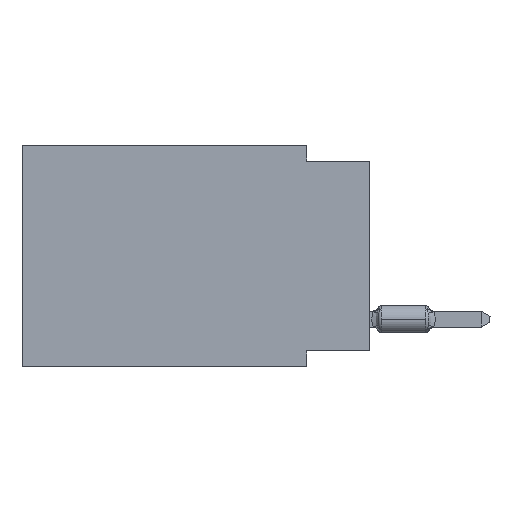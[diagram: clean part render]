
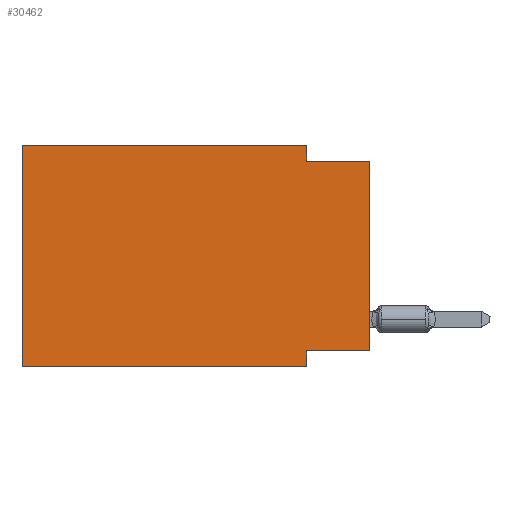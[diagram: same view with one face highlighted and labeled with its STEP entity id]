
A CAD part, left-side view. The second image highlights one B-rep face of the part: STEP entity #30462.
In plain terms, the highlighted planar face has unit normal (-1, 0, 0).
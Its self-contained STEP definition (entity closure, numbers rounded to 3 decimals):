
#1430 = VERTEX_POINT ( 'NONE', #4107 ) ;
#1948 = ORIENTED_EDGE ( 'NONE', *, *, #29080, .F. ) ;
#2856 = ORIENTED_EDGE ( 'NONE', *, *, #14217, .F. ) ;
#3091 = CARTESIAN_POINT ( 'NONE',  ( 0., 2.54, 0. ) ) ;
#3257 = DIRECTION ( 'NONE',  ( 1., 0., 0. ) ) ;
#3844 = VERTEX_POINT ( 'NONE', #28738 ) ;
#4045 = EDGE_CURVE ( 'NONE', #5214, #22583, #24029, .T. ) ;
#4107 = CARTESIAN_POINT ( 'NONE',  ( 0., 2.54, -8.255 ) ) ;
#5006 = DIRECTION ( 'NONE',  ( 0., -1., 0. ) ) ;
#5214 = VERTEX_POINT ( 'NONE', #34189 ) ;
#6001 = VECTOR ( 'NONE', #5006, 1000. ) ;
#6432 = VERTEX_POINT ( 'NONE', #11158 ) ;
#7001 = LINE ( 'NONE', #20782, #9131 ) ;
#7038 = AXIS2_PLACEMENT_3D ( 'NONE', #30277, #3257, #16506 ) ;
#7284 = CARTESIAN_POINT ( 'NONE',  ( 0., 0., -0.635 ) ) ;
#7659 = CARTESIAN_POINT ( 'NONE',  ( 0., 13.97, 0. ) ) ;
#8152 = DIRECTION ( 'NONE',  ( 0., 0., -1. ) ) ;
#9131 = VECTOR ( 'NONE', #31422, 1000. ) ;
#10201 = VECTOR ( 'NONE', #8152, 1000. ) ;
#10367 = DIRECTION ( 'NONE',  ( 0., 0., -1. ) ) ;
#10886 = ORIENTED_EDGE ( 'NONE', *, *, #30769, .F. ) ;
#11158 = CARTESIAN_POINT ( 'NONE',  ( 0., 2.54, -8.89 ) ) ;
#11783 = CARTESIAN_POINT ( 'NONE',  ( 0., 0., -8.255 ) ) ;
#13249 = CARTESIAN_POINT ( 'NONE',  ( 0., 2.54, -0.635 ) ) ;
#14217 = EDGE_CURVE ( 'NONE', #19868, #3844, #7001, .T. ) ;
#14917 = CARTESIAN_POINT ( 'NONE',  ( 0., 13.97, -8.89 ) ) ;
#15232 = VERTEX_POINT ( 'NONE', #20345 ) ;
#15614 = CARTESIAN_POINT ( 'NONE',  ( 0., 2.54, -8.89 ) ) ;
#16506 = DIRECTION ( 'NONE',  ( 0., 0., -1. ) ) ;
#16698 = DIRECTION ( 'NONE',  ( 0., 1., 0. ) ) ;
#16873 = VECTOR ( 'NONE', #20662, 1000. ) ;
#16999 = VECTOR ( 'NONE', #10367, 1000. ) ;
#17477 = VECTOR ( 'NONE', #30447, 1000. ) ;
#17863 = CARTESIAN_POINT ( 'NONE',  ( 0., 0., 0. ) ) ;
#18821 = DIRECTION ( 'NONE',  ( 0., -1., 0. ) ) ;
#19123 = PLANE ( 'NONE',  #7038 ) ;
#19319 = LINE ( 'NONE', #29962, #30043 ) ;
#19769 = ORIENTED_EDGE ( 'NONE', *, *, #19881, .F. ) ;
#19868 = VERTEX_POINT ( 'NONE', #21770 ) ;
#19881 = EDGE_CURVE ( 'NONE', #31110, #1430, #19319, .T. ) ;
#20130 = ORIENTED_EDGE ( 'NONE', *, *, #4045, .F. ) ;
#20338 = ORIENTED_EDGE ( 'NONE', *, *, #28699, .F. ) ;
#20345 = CARTESIAN_POINT ( 'NONE',  ( 0., 0., -0.635 ) ) ;
#20662 = DIRECTION ( 'NONE',  ( 0., 0., 1. ) ) ;
#20782 = CARTESIAN_POINT ( 'NONE',  ( 0., 13.97, 0. ) ) ;
#21611 = LINE ( 'NONE', #7659, #30908 ) ;
#21770 = CARTESIAN_POINT ( 'NONE',  ( 0., 13.97, -8.89 ) ) ;
#21906 = FACE_OUTER_BOUND ( 'NONE', #30085, .T. ) ;
#22583 = VERTEX_POINT ( 'NONE', #13249 ) ;
#24029 = LINE ( 'NONE', #3091, #10201 ) ;
#24953 = EDGE_CURVE ( 'NONE', #31110, #15232, #28504, .T. ) ;
#25897 = EDGE_CURVE ( 'NONE', #19868, #6432, #31139, .T. ) ;
#26067 = LINE ( 'NONE', #15614, #16999 ) ;
#28504 = LINE ( 'NONE', #17863, #16873 ) ;
#28699 = EDGE_CURVE ( 'NONE', #3844, #5214, #21611, .T. ) ;
#28738 = CARTESIAN_POINT ( 'NONE',  ( 0., 13.97, 0. ) ) ;
#28912 = LINE ( 'NONE', #7284, #6001 ) ;
#29080 = EDGE_CURVE ( 'NONE', #1430, #6432, #26067, .T. ) ;
#29962 = CARTESIAN_POINT ( 'NONE',  ( 0., 0., -8.255 ) ) ;
#30043 = VECTOR ( 'NONE', #16698, 1000. ) ;
#30085 = EDGE_LOOP ( 'NONE', ( #32692, #10886, #20130, #20338, #2856, #30700, #1948, #19769 ) ) ;
#30277 = CARTESIAN_POINT ( 'NONE',  ( 0., 13.97, 0. ) ) ;
#30447 = DIRECTION ( 'NONE',  ( 0., -1., 0. ) ) ;
#30462 = ADVANCED_FACE ( 'NONE', ( #21906 ), #19123, .F. ) ;
#30700 = ORIENTED_EDGE ( 'NONE', *, *, #25897, .T. ) ;
#30769 = EDGE_CURVE ( 'NONE', #22583, #15232, #28912, .T. ) ;
#30908 = VECTOR ( 'NONE', #18821, 1000. ) ;
#31110 = VERTEX_POINT ( 'NONE', #11783 ) ;
#31139 = LINE ( 'NONE', #14917, #17477 ) ;
#31422 = DIRECTION ( 'NONE',  ( 0., 0., 1. ) ) ;
#32692 = ORIENTED_EDGE ( 'NONE', *, *, #24953, .T. ) ;
#34189 = CARTESIAN_POINT ( 'NONE',  ( 0., 2.54, 0. ) ) ;
